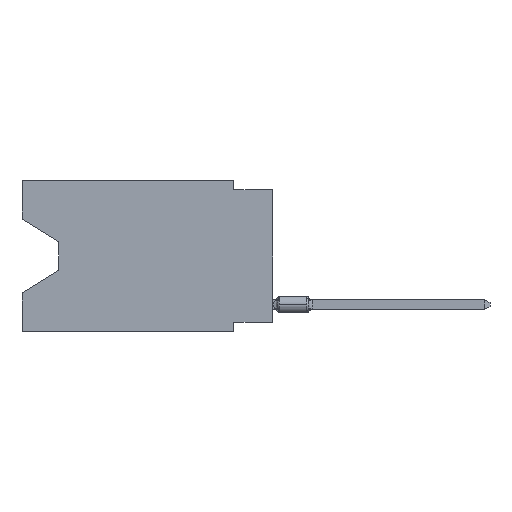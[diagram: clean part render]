
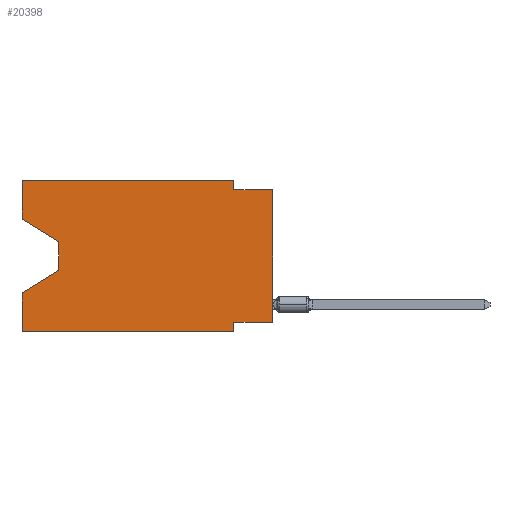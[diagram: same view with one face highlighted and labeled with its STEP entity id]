
A CAD part, left-side view. The second image highlights one B-rep face of the part: STEP entity #20398.
In plain terms, the highlighted planar face has unit normal (-1, 0, 0).
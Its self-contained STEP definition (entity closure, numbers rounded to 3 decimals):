
#47 = LINE ( 'NONE', #22705, #22554 ) ;
#63 = CARTESIAN_POINT ( 'NONE',  ( 0., 13.97, -4.013 ) ) ;
#231 = CARTESIAN_POINT ( 'NONE',  ( 0., 16.383, 0. ) ) ;
#506 = EDGE_CURVE ( 'NONE', #4507, #6325, #4874, .T. ) ;
#539 = VERTEX_POINT ( 'NONE', #7433 ) ;
#604 = ORIENTED_EDGE ( 'NONE', *, *, #16129, .F. ) ;
#636 = ORIENTED_EDGE ( 'NONE', *, *, #9146, .F. ) ;
#901 = CARTESIAN_POINT ( 'NONE',  ( 0., 13.97, -5.893 ) ) ;
#1114 = ORIENTED_EDGE ( 'NONE', *, *, #4111, .F. ) ;
#1229 = EDGE_CURVE ( 'NONE', #24948, #15011, #2037, .T. ) ;
#1522 = VECTOR ( 'NONE', #7067, 1000. ) ;
#1658 = EDGE_CURVE ( 'NONE', #6325, #18844, #23377, .T. ) ;
#2037 = LINE ( 'NONE', #11732, #22465 ) ;
#2216 = CARTESIAN_POINT ( 'NONE',  ( 0., 16.383, -2.546 ) ) ;
#2291 = EDGE_CURVE ( 'NONE', #6624, #23696, #4620, .T. ) ;
#2529 = VECTOR ( 'NONE', #15197, 1000. ) ;
#2602 = VECTOR ( 'NONE', #20150, 1000. ) ;
#2743 = CARTESIAN_POINT ( 'NONE',  ( 0., 2.54, -0.635 ) ) ;
#4111 = EDGE_CURVE ( 'NONE', #24948, #12536, #47, .T. ) ;
#4415 = DIRECTION ( 'NONE',  ( 0., 0., -1. ) ) ;
#4422 = ORIENTED_EDGE ( 'NONE', *, *, #14086, .F. ) ;
#4507 = VERTEX_POINT ( 'NONE', #9882 ) ;
#4620 = LINE ( 'NONE', #12401, #2602 ) ;
#4621 = EDGE_CURVE ( 'NONE', #13453, #539, #12915, .T. ) ;
#4874 = LINE ( 'NONE', #24721, #2529 ) ;
#5813 = EDGE_CURVE ( 'NONE', #17391, #17931, #17376, .T. ) ;
#5834 = VECTOR ( 'NONE', #7866, 1000. ) ;
#6303 = VECTOR ( 'NONE', #9634, 1000. ) ;
#6325 = VERTEX_POINT ( 'NONE', #10559 ) ;
#6538 = ORIENTED_EDGE ( 'NONE', *, *, #1658, .F. ) ;
#6624 = VERTEX_POINT ( 'NONE', #15867 ) ;
#7066 = VECTOR ( 'NONE', #4415, 1000. ) ;
#7067 = DIRECTION ( 'NONE',  ( 0., 0., 1. ) ) ;
#7392 = LINE ( 'NONE', #23272, #8412 ) ;
#7433 = CARTESIAN_POINT ( 'NONE',  ( 0., 16.383, -7.36 ) ) ;
#7866 = DIRECTION ( 'NONE',  ( 0., 0., 1. ) ) ;
#7984 = CARTESIAN_POINT ( 'NONE',  ( 0., 2.54, -9.906 ) ) ;
#8102 = ORIENTED_EDGE ( 'NONE', *, *, #4621, .T. ) ;
#8391 = VECTOR ( 'NONE', #18703, 1000. ) ;
#8412 = VECTOR ( 'NONE', #15029, 1000. ) ;
#9146 = EDGE_CURVE ( 'NONE', #12536, #23696, #16279, .T. ) ;
#9634 = DIRECTION ( 'NONE',  ( 0., -0.855, -0.519 ) ) ;
#9882 = CARTESIAN_POINT ( 'NONE',  ( 0., 16.383, 0. ) ) ;
#10020 = ORIENTED_EDGE ( 'NONE', *, *, #24813, .T. ) ;
#10559 = CARTESIAN_POINT ( 'NONE',  ( 0., 2.54, 0. ) ) ;
#10620 = DIRECTION ( 'NONE',  ( 0., 0., -1. ) ) ;
#10636 = CARTESIAN_POINT ( 'NONE',  ( 0., 16.383, 0. ) ) ;
#11016 = LINE ( 'NONE', #10636, #1522 ) ;
#11732 = CARTESIAN_POINT ( 'NONE',  ( 0., 0., 0. ) ) ;
#12401 = CARTESIAN_POINT ( 'NONE',  ( 0., 16.383, -9.906 ) ) ;
#12536 = VERTEX_POINT ( 'NONE', #16484 ) ;
#12915 = LINE ( 'NONE', #18355, #25035 ) ;
#13453 = VERTEX_POINT ( 'NONE', #901 ) ;
#13846 = CARTESIAN_POINT ( 'NONE',  ( 0., 2.54, 0. ) ) ;
#13992 = ORIENTED_EDGE ( 'NONE', *, *, #24996, .F. ) ;
#14086 = EDGE_CURVE ( 'NONE', #17391, #4507, #17897, .T. ) ;
#14445 = DIRECTION ( 'NONE',  ( 1., 0., 0. ) ) ;
#15011 = VERTEX_POINT ( 'NONE', #16012 ) ;
#15029 = DIRECTION ( 'NONE',  ( 0., -1., 0. ) ) ;
#15147 = LINE ( 'NONE', #16800, #8391 ) ;
#15197 = DIRECTION ( 'NONE',  ( 0., -1., 0. ) ) ;
#15602 = ORIENTED_EDGE ( 'NONE', *, *, #506, .F. ) ;
#15867 = CARTESIAN_POINT ( 'NONE',  ( 0., 16.383, -9.906 ) ) ;
#16012 = CARTESIAN_POINT ( 'NONE',  ( 0., 0., -0.635 ) ) ;
#16034 = DIRECTION ( 'NONE',  ( 0., 0., -1. ) ) ;
#16129 = EDGE_CURVE ( 'NONE', #18844, #15011, #7392, .T. ) ;
#16279 = LINE ( 'NONE', #16545, #17872 ) ;
#16457 = CARTESIAN_POINT ( 'NONE',  ( 0., 16.383, 0. ) ) ;
#16484 = CARTESIAN_POINT ( 'NONE',  ( 0., 2.54, -9.271 ) ) ;
#16545 = CARTESIAN_POINT ( 'NONE',  ( 0., 2.54, -9.906 ) ) ;
#16800 = CARTESIAN_POINT ( 'NONE',  ( 0., 13.97, -4.013 ) ) ;
#17376 = LINE ( 'NONE', #2216, #6303 ) ;
#17391 = VERTEX_POINT ( 'NONE', #20768 ) ;
#17872 = VECTOR ( 'NONE', #16034, 1000. ) ;
#17897 = LINE ( 'NONE', #231, #5834 ) ;
#17931 = VERTEX_POINT ( 'NONE', #63 ) ;
#17995 = EDGE_LOOP ( 'NONE', ( #24099, #10020, #8102, #13992, #22287, #636, #1114, #24427, #604, #6538, #15602, #4422 ) ) ;
#18116 = FACE_OUTER_BOUND ( 'NONE', #17995, .T. ) ;
#18355 = CARTESIAN_POINT ( 'NONE',  ( 0., 13.97, -5.893 ) ) ;
#18703 = DIRECTION ( 'NONE',  ( 0., 0., -1. ) ) ;
#18844 = VERTEX_POINT ( 'NONE', #2743 ) ;
#19671 = AXIS2_PLACEMENT_3D ( 'NONE', #16457, #14445, #10620 ) ;
#20150 = DIRECTION ( 'NONE',  ( 0., -1., 0. ) ) ;
#20398 = ADVANCED_FACE ( 'NONE', ( #18116 ), #21917, .F. ) ;
#20650 = DIRECTION ( 'NONE',  ( 0., 0.855, -0.519 ) ) ;
#20681 = DIRECTION ( 'NONE',  ( 0., 1., 0. ) ) ;
#20768 = CARTESIAN_POINT ( 'NONE',  ( 0., 16.383, -2.546 ) ) ;
#21917 = PLANE ( 'NONE',  #19671 ) ;
#22287 = ORIENTED_EDGE ( 'NONE', *, *, #2291, .T. ) ;
#22465 = VECTOR ( 'NONE', #23902, 1000. ) ;
#22554 = VECTOR ( 'NONE', #20681, 1000. ) ;
#22705 = CARTESIAN_POINT ( 'NONE',  ( 0., 0., -9.271 ) ) ;
#23272 = CARTESIAN_POINT ( 'NONE',  ( 0., 0., -0.635 ) ) ;
#23377 = LINE ( 'NONE', #13846, #7066 ) ;
#23696 = VERTEX_POINT ( 'NONE', #7984 ) ;
#23902 = DIRECTION ( 'NONE',  ( 0., 0., 1. ) ) ;
#24099 = ORIENTED_EDGE ( 'NONE', *, *, #5813, .T. ) ;
#24427 = ORIENTED_EDGE ( 'NONE', *, *, #1229, .T. ) ;
#24471 = CARTESIAN_POINT ( 'NONE',  ( 0., 0., -9.271 ) ) ;
#24721 = CARTESIAN_POINT ( 'NONE',  ( 0., 16.383, 0. ) ) ;
#24813 = EDGE_CURVE ( 'NONE', #17931, #13453, #15147, .T. ) ;
#24948 = VERTEX_POINT ( 'NONE', #24471 ) ;
#24996 = EDGE_CURVE ( 'NONE', #6624, #539, #11016, .T. ) ;
#25035 = VECTOR ( 'NONE', #20650, 1000. ) ;
